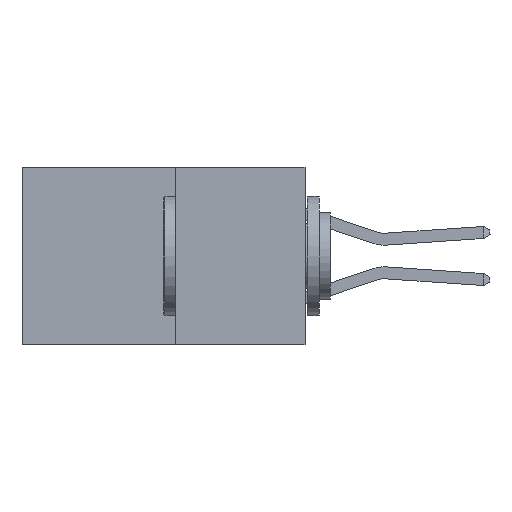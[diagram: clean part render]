
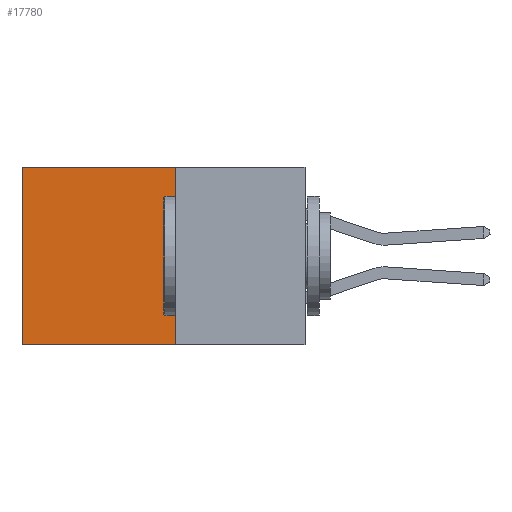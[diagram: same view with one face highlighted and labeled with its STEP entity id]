
A CAD part, left-side view. The second image highlights one B-rep face of the part: STEP entity #17780.
In plain terms, the highlighted planar face has unit normal (-1, 0, 0).
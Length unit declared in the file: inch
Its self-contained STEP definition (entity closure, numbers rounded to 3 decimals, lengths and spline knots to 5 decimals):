
#517 = VERTEX_POINT ( 'NONE', #16365 ) ;
#830 = DIRECTION ( 'NONE',  ( 1., 0., 0. ) ) ;
#1291 = VECTOR ( 'NONE', #3109, 39.37008 ) ;
#1401 = CARTESIAN_POINT ( 'NONE',  ( 0.277, 0.27, -0.37 ) ) ;
#1596 = CARTESIAN_POINT ( 'NONE',  ( 0.277, 0.27, -0.37 ) ) ;
#2140 = AXIS2_PLACEMENT_3D ( 'NONE', #9441, #830, #10840 ) ;
#2891 = LINE ( 'NONE', #11999, #17449 ) ;
#3109 = DIRECTION ( 'NONE',  ( 0., 1., 0. ) ) ;
#6601 = VERTEX_POINT ( 'NONE', #18337 ) ;
#6931 = FACE_OUTER_BOUND ( 'NONE', #8859, .T. ) ;
#6944 = VECTOR ( 'NONE', #18291, 39.37008 ) ;
#7486 = VECTOR ( 'NONE', #12890, 39.37008 ) ;
#8413 = EDGE_CURVE ( 'NONE', #15775, #18269, #2891, .T. ) ;
#8786 = ORIENTED_EDGE ( 'NONE', *, *, #16685, .T. ) ;
#8859 = EDGE_LOOP ( 'NONE', ( #8786, #14395, #16814, #18012 ) ) ;
#8904 = LINE ( 'NONE', #1596, #1291 ) ;
#9441 = CARTESIAN_POINT ( 'NONE',  ( 0.277, 0.27, -0.37 ) ) ;
#10420 = EDGE_CURVE ( 'NONE', #15775, #517, #11256, .T. ) ;
#10669 = LINE ( 'NONE', #11317, #6944 ) ;
#10840 = DIRECTION ( 'NONE',  ( 0., 0., -1. ) ) ;
#10844 = CARTESIAN_POINT ( 'NONE',  ( 0.277, 0.27, 0. ) ) ;
#11256 = LINE ( 'NONE', #1401, #7486 ) ;
#11317 = CARTESIAN_POINT ( 'NONE',  ( 0.277, 0.59, -0.37 ) ) ;
#11999 = CARTESIAN_POINT ( 'NONE',  ( 0.277, 0.27, 0. ) ) ;
#12890 = DIRECTION ( 'NONE',  ( 0., 0., -1. ) ) ;
#14395 = ORIENTED_EDGE ( 'NONE', *, *, #16787, .F. ) ;
#14910 = DIRECTION ( 'NONE',  ( 0., 1., 0. ) ) ;
#15775 = VERTEX_POINT ( 'NONE', #10844 ) ;
#16365 = CARTESIAN_POINT ( 'NONE',  ( 0.277, 0.27, -0.37 ) ) ;
#16685 = EDGE_CURVE ( 'NONE', #18269, #6601, #10669, .T. ) ;
#16787 = EDGE_CURVE ( 'NONE', #517, #6601, #8904, .T. ) ;
#16814 = ORIENTED_EDGE ( 'NONE', *, *, #10420, .F. ) ;
#17413 = CARTESIAN_POINT ( 'NONE',  ( 0.277, 0.59, 0. ) ) ;
#17449 = VECTOR ( 'NONE', #14910, 39.37008 ) ;
#17780 = ADVANCED_FACE ( 'NONE', ( #6931 ), #17825, .F. ) ;
#17825 = PLANE ( 'NONE',  #2140 ) ;
#18012 = ORIENTED_EDGE ( 'NONE', *, *, #8413, .T. ) ;
#18269 = VERTEX_POINT ( 'NONE', #17413 ) ;
#18291 = DIRECTION ( 'NONE',  ( 0., 0., -1. ) ) ;
#18337 = CARTESIAN_POINT ( 'NONE',  ( 0.277, 0.59, -0.37 ) ) ;
